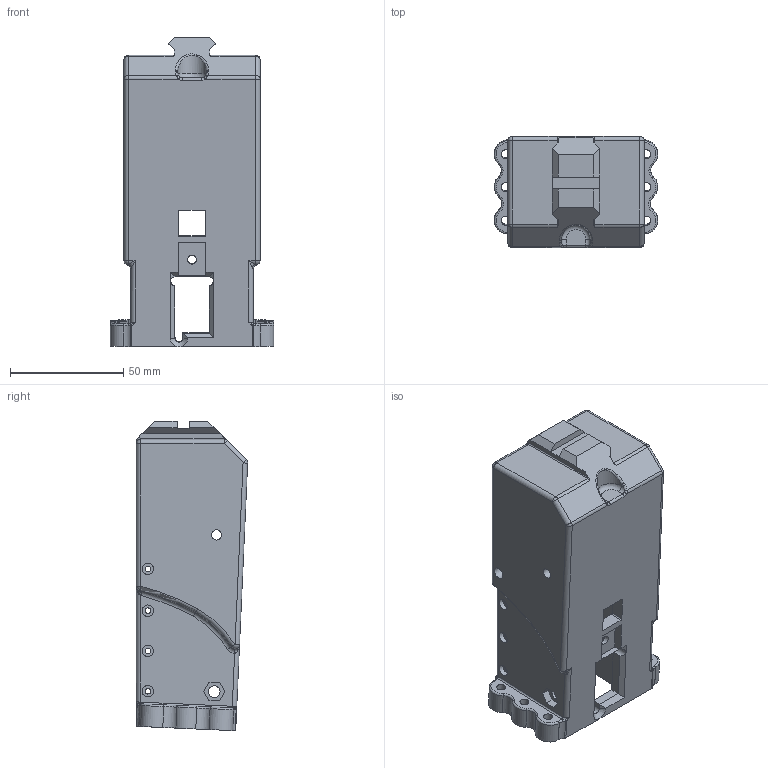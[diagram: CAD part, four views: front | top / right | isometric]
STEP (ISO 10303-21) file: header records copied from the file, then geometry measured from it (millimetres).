
FILE_DESCRIPTION(/* description */ (''),/* implementation_level */ '2;1');
FILE_NAME(/* name */ 'Plastikov v3.1 Rear Receiver Pic Rail Rear End.stp',/* time_stamp */ '2022-03-25T09:33:41-05:00',/* author */ ('johne'),/* organization */ (''),/* preprocessor_version */ 'ST-DEVELOPER v18.1',/* originating_system */ 'Autodesk Inventor 2020',/* authorisation */ '');
FILE_SCHEMA (('AUTOMOTIVE_DESIGN { 1 0 10303 214 3 1 1 }','TECHNICAL_DATA_PACKAGING'));
Products named in the file (1): Plastikov v3.1 Rear Receiver AR15 Stock
Bounding box: 72.2 x 49.14 x 136.76 mm (x, y, z)
Volume: 213135.1 mm3; surface area: 44475.5 mm2
Topology: 1 solids, 15 shells, 319 faces, 751 edges, 461 vertices
Faces by surface type: plane 105, cylinder 98, bspline 64, torus 35, sphere 16, cone 1
Full cylindrical faces by diameter (mm): 2.5 x8, 4 x7, 4.5 x2, 5.08 x8, 5.1 x2, 12 x1
Entity records: 34459 total; most frequent: CARTESIAN_POINT 26993, ORIENTED_EDGE 1482, DIRECTION 1471, EDGE_CURVE 741, AXIS2_PLACEMENT_3D 578, VERTEX_POINT 461, EDGE_LOOP 370, FACE_OUTER_BOUND 319
